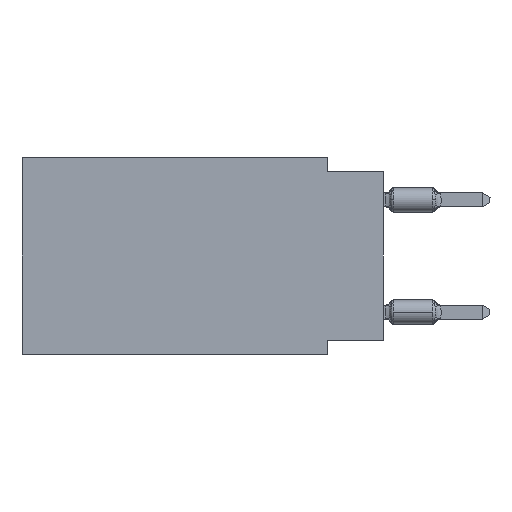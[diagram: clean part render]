
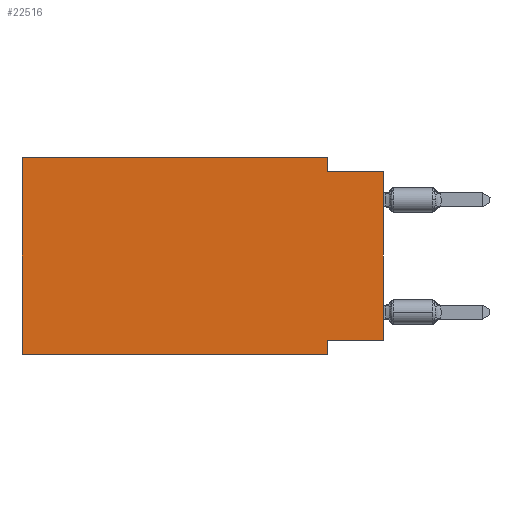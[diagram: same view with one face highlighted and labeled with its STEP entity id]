
A CAD part, left-side view. The second image highlights one B-rep face of the part: STEP entity #22516.
In plain terms, the highlighted planar face has unit normal (-1, 0, 0).
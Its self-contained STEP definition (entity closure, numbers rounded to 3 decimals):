
#547 = EDGE_CURVE ( 'NONE', #5898, #22962, #34979, .T. ) ;
#1069 = VERTEX_POINT ( 'NONE', #22340 ) ;
#1139 = ORIENTED_EDGE ( 'NONE', *, *, #28084, .T. ) ;
#1404 = DIRECTION ( 'NONE',  ( 0., 0., -1. ) ) ;
#1584 = VERTEX_POINT ( 'NONE', #26498 ) ;
#1588 = CARTESIAN_POINT ( 'NONE',  ( 0., 16.383, 0. ) ) ;
#1877 = VECTOR ( 'NONE', #5906, 1000. ) ;
#3932 = ORIENTED_EDGE ( 'NONE', *, *, #547, .F. ) ;
#4757 = CARTESIAN_POINT ( 'NONE',  ( 0., 0., -0.635 ) ) ;
#5338 = LINE ( 'NONE', #26572, #1877 ) ;
#5356 = CARTESIAN_POINT ( 'NONE',  ( 0., 0., -8.255 ) ) ;
#5898 = VERTEX_POINT ( 'NONE', #37028 ) ;
#5906 = DIRECTION ( 'NONE',  ( 0., 0., 1. ) ) ;
#5934 = ORIENTED_EDGE ( 'NONE', *, *, #23776, .F. ) ;
#6565 = ORIENTED_EDGE ( 'NONE', *, *, #21603, .T. ) ;
#6913 = DIRECTION ( 'NONE',  ( 0., 0., 1. ) ) ;
#8499 = DIRECTION ( 'NONE',  ( 0., -1., 0. ) ) ;
#9049 = VERTEX_POINT ( 'NONE', #27299 ) ;
#9386 = EDGE_CURVE ( 'NONE', #14355, #12565, #15972, .T. ) ;
#9436 = VECTOR ( 'NONE', #19584, 1000. ) ;
#9492 = LINE ( 'NONE', #33076, #12910 ) ;
#9533 = EDGE_CURVE ( 'NONE', #23165, #1584, #19662, .T. ) ;
#9784 = LINE ( 'NONE', #24314, #21658 ) ;
#11789 = VECTOR ( 'NONE', #24313, 1000. ) ;
#12565 = VERTEX_POINT ( 'NONE', #4757 ) ;
#12910 = VECTOR ( 'NONE', #29585, 1000. ) ;
#12995 = DIRECTION ( 'NONE',  ( 1., 0., 0. ) ) ;
#14355 = VERTEX_POINT ( 'NONE', #32462 ) ;
#14508 = CARTESIAN_POINT ( 'NONE',  ( 0., 16.383, 0. ) ) ;
#15168 = EDGE_CURVE ( 'NONE', #9049, #5898, #5338, .T. ) ;
#15887 = LINE ( 'NONE', #19408, #9436 ) ;
#15972 = LINE ( 'NONE', #33394, #31289 ) ;
#16084 = FACE_OUTER_BOUND ( 'NONE', #31344, .T. ) ;
#16250 = ORIENTED_EDGE ( 'NONE', *, *, #9533, .F. ) ;
#16791 = AXIS2_PLACEMENT_3D ( 'NONE', #1588, #12995, #1404 ) ;
#19408 = CARTESIAN_POINT ( 'NONE',  ( 0., 2.54, 0. ) ) ;
#19584 = DIRECTION ( 'NONE',  ( 0., 0., -1. ) ) ;
#19662 = LINE ( 'NONE', #37272, #37497 ) ;
#21603 = EDGE_CURVE ( 'NONE', #9049, #1069, #27395, .T. ) ;
#21658 = VECTOR ( 'NONE', #6913, 1000. ) ;
#21797 = VECTOR ( 'NONE', #8499, 1000. ) ;
#22175 = DIRECTION ( 'NONE',  ( 0., 1., 0. ) ) ;
#22340 = CARTESIAN_POINT ( 'NONE',  ( 0., 2.54, -8.89 ) ) ;
#22516 = ADVANCED_FACE ( 'NONE', ( #16084 ), #27880, .F. ) ;
#22962 = VERTEX_POINT ( 'NONE', #28345 ) ;
#23165 = VERTEX_POINT ( 'NONE', #5356 ) ;
#23776 = EDGE_CURVE ( 'NONE', #22962, #14355, #15887, .T. ) ;
#24313 = DIRECTION ( 'NONE',  ( 0., -1., 0. ) ) ;
#24314 = CARTESIAN_POINT ( 'NONE',  ( 0., 0., 0. ) ) ;
#24677 = CARTESIAN_POINT ( 'NONE',  ( 0., 16.383, -8.89 ) ) ;
#25144 = ORIENTED_EDGE ( 'NONE', *, *, #15168, .F. ) ;
#26483 = ORIENTED_EDGE ( 'NONE', *, *, #9386, .F. ) ;
#26498 = CARTESIAN_POINT ( 'NONE',  ( 0., 2.54, -8.255 ) ) ;
#26572 = CARTESIAN_POINT ( 'NONE',  ( 0., 16.383, 0. ) ) ;
#27299 = CARTESIAN_POINT ( 'NONE',  ( 0., 16.383, -8.89 ) ) ;
#27395 = LINE ( 'NONE', #24677, #11789 ) ;
#27880 = PLANE ( 'NONE',  #16791 ) ;
#28084 = EDGE_CURVE ( 'NONE', #23165, #12565, #9784, .T. ) ;
#28345 = CARTESIAN_POINT ( 'NONE',  ( 0., 2.54, 0. ) ) ;
#29585 = DIRECTION ( 'NONE',  ( 0., 0., -1. ) ) ;
#30418 = ORIENTED_EDGE ( 'NONE', *, *, #34685, .F. ) ;
#31289 = VECTOR ( 'NONE', #36684, 1000. ) ;
#31344 = EDGE_LOOP ( 'NONE', ( #1139, #26483, #5934, #3932, #25144, #6565, #30418, #16250 ) ) ;
#32462 = CARTESIAN_POINT ( 'NONE',  ( 0., 2.54, -0.635 ) ) ;
#33076 = CARTESIAN_POINT ( 'NONE',  ( 0., 2.54, -8.89 ) ) ;
#33394 = CARTESIAN_POINT ( 'NONE',  ( 0., 0., -0.635 ) ) ;
#34685 = EDGE_CURVE ( 'NONE', #1584, #1069, #9492, .T. ) ;
#34979 = LINE ( 'NONE', #14508, #21797 ) ;
#36684 = DIRECTION ( 'NONE',  ( 0., -1., 0. ) ) ;
#37028 = CARTESIAN_POINT ( 'NONE',  ( 0., 16.383, 0. ) ) ;
#37272 = CARTESIAN_POINT ( 'NONE',  ( 0., 0., -8.255 ) ) ;
#37497 = VECTOR ( 'NONE', #22175, 1000. ) ;
